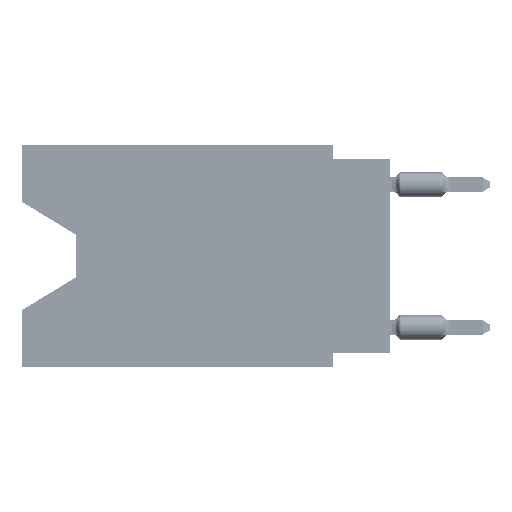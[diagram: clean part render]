
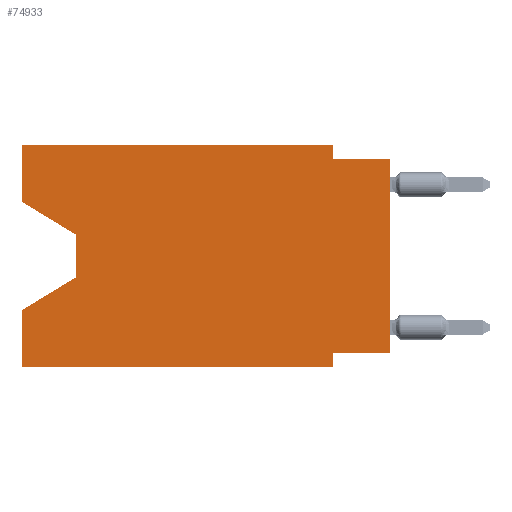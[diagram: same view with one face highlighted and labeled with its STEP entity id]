
A CAD part, left-side view. The second image highlights one B-rep face of the part: STEP entity #74933.
In plain terms, the highlighted planar face has unit normal (-1, 0, 0).
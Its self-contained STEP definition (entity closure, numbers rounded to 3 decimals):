
#1643 = ORIENTED_EDGE ( 'NONE', *, *, #59581, .T. ) ;
#3767 = CARTESIAN_POINT ( 'NONE',  ( 0., 13.97, -4.013 ) ) ;
#3869 = CARTESIAN_POINT ( 'NONE',  ( 0., 13.97, -5.893 ) ) ;
#3944 = VERTEX_POINT ( 'NONE', #62409 ) ;
#4007 = VERTEX_POINT ( 'NONE', #27999 ) ;
#4010 = VECTOR ( 'NONE', #70191, 1000. ) ;
#4307 = ORIENTED_EDGE ( 'NONE', *, *, #34257, .T. ) ;
#4495 = ORIENTED_EDGE ( 'NONE', *, *, #72244, .F. ) ;
#5738 = DIRECTION ( 'NONE',  ( 0., 1., 0. ) ) ;
#5944 = ORIENTED_EDGE ( 'NONE', *, *, #39216, .T. ) ;
#6484 = CARTESIAN_POINT ( 'NONE',  ( 0., 0., -9.271 ) ) ;
#7124 = ORIENTED_EDGE ( 'NONE', *, *, #42013, .F. ) ;
#7184 = PLANE ( 'NONE',  #61906 ) ;
#7588 = VECTOR ( 'NONE', #34961, 1000. ) ;
#7641 = DIRECTION ( 'NONE',  ( 0., -0.855, -0.519 ) ) ;
#9829 = VECTOR ( 'NONE', #7641, 1000. ) ;
#9914 = VERTEX_POINT ( 'NONE', #3767 ) ;
#10102 = ORIENTED_EDGE ( 'NONE', *, *, #59557, .F. ) ;
#10778 = CARTESIAN_POINT ( 'NONE',  ( 0., 2.54, -9.271 ) ) ;
#11284 = EDGE_CURVE ( 'NONE', #56904, #65937, #42937, .T. ) ;
#11451 = CARTESIAN_POINT ( 'NONE',  ( 0., 2.54, 0. ) ) ;
#12193 = ORIENTED_EDGE ( 'NONE', *, *, #66778, .F. ) ;
#13023 = DIRECTION ( 'NONE',  ( 0., -1., 0. ) ) ;
#14417 = CARTESIAN_POINT ( 'NONE',  ( 0., 16.383, 0. ) ) ;
#15063 = CARTESIAN_POINT ( 'NONE',  ( 0., 16.383, 0. ) ) ;
#16165 = LINE ( 'NONE', #58959, #32731 ) ;
#17858 = LINE ( 'NONE', #11451, #47762 ) ;
#19042 = LINE ( 'NONE', #67795, #57988 ) ;
#21041 = DIRECTION ( 'NONE',  ( 0., -1., 0. ) ) ;
#22310 = CARTESIAN_POINT ( 'NONE',  ( 0., 2.54, 0. ) ) ;
#24592 = VERTEX_POINT ( 'NONE', #46143 ) ;
#24802 = DIRECTION ( 'NONE',  ( 0., 0., -1. ) ) ;
#24850 = VERTEX_POINT ( 'NONE', #26475 ) ;
#25269 = VERTEX_POINT ( 'NONE', #62284 ) ;
#26475 = CARTESIAN_POINT ( 'NONE',  ( 0., 16.383, -2.546 ) ) ;
#27052 = EDGE_CURVE ( 'NONE', #24850, #25269, #40960, .T. ) ;
#27944 = CARTESIAN_POINT ( 'NONE',  ( 0., 0., -0.635 ) ) ;
#27999 = CARTESIAN_POINT ( 'NONE',  ( 0., 0., -0.635 ) ) ;
#28840 = CARTESIAN_POINT ( 'NONE',  ( 0., 2.54, -9.906 ) ) ;
#30872 = VERTEX_POINT ( 'NONE', #74119 ) ;
#31520 = CARTESIAN_POINT ( 'NONE',  ( 0., 13.97, -4.013 ) ) ;
#32284 = LINE ( 'NONE', #15063, #56442 ) ;
#32670 = LINE ( 'NONE', #31520, #69686 ) ;
#32731 = VECTOR ( 'NONE', #70539, 1000. ) ;
#32813 = ORIENTED_EDGE ( 'NONE', *, *, #77363, .T. ) ;
#32839 = LINE ( 'NONE', #14417, #78806 ) ;
#33634 = VERTEX_POINT ( 'NONE', #28840 ) ;
#34257 = EDGE_CURVE ( 'NONE', #9914, #63032, #32670, .T. ) ;
#34961 = DIRECTION ( 'NONE',  ( 0., 0., 1. ) ) ;
#35899 = VERTEX_POINT ( 'NONE', #22310 ) ;
#36657 = DIRECTION ( 'NONE',  ( 0., 0., -1. ) ) ;
#36780 = ORIENTED_EDGE ( 'NONE', *, *, #63275, .F. ) ;
#37490 = VECTOR ( 'NONE', #5738, 1000. ) ;
#38815 = DIRECTION ( 'NONE',  ( 0., 0., 1. ) ) ;
#39216 = EDGE_CURVE ( 'NONE', #63032, #24592, #58665, .T. ) ;
#40960 = LINE ( 'NONE', #65336, #7588 ) ;
#42013 = EDGE_CURVE ( 'NONE', #25269, #35899, #32284, .T. ) ;
#42151 = VECTOR ( 'NONE', #69914, 1000. ) ;
#42937 = LINE ( 'NONE', #66529, #37490 ) ;
#46143 = CARTESIAN_POINT ( 'NONE',  ( 0., 16.383, -7.36 ) ) ;
#46328 = LINE ( 'NONE', #27944, #42151 ) ;
#47762 = VECTOR ( 'NONE', #36657, 1000. ) ;
#49720 = EDGE_CURVE ( 'NONE', #3944, #33634, #19042, .T. ) ;
#55583 = FACE_OUTER_BOUND ( 'NONE', #58093, .T. ) ;
#56442 = VECTOR ( 'NONE', #21041, 1000. ) ;
#56891 = ORIENTED_EDGE ( 'NONE', *, *, #49720, .T. ) ;
#56904 = VERTEX_POINT ( 'NONE', #6484 ) ;
#57058 = DIRECTION ( 'NONE',  ( 0., 0., -1. ) ) ;
#57231 = CARTESIAN_POINT ( 'NONE',  ( 0., 16.383, -2.546 ) ) ;
#57988 = VECTOR ( 'NONE', #13023, 1000. ) ;
#58093 = EDGE_LOOP ( 'NONE', ( #1643, #4307, #5944, #10102, #56891, #12193, #66478, #32813, #36780, #4495, #7124, #60650 ) ) ;
#58213 = CARTESIAN_POINT ( 'NONE',  ( 0., 2.54, -9.906 ) ) ;
#58665 = LINE ( 'NONE', #3869, #73938 ) ;
#58959 = CARTESIAN_POINT ( 'NONE',  ( 0., 0., 0. ) ) ;
#59557 = EDGE_CURVE ( 'NONE', #3944, #24592, #32839, .T. ) ;
#59581 = EDGE_CURVE ( 'NONE', #24850, #9914, #62056, .T. ) ;
#60650 = ORIENTED_EDGE ( 'NONE', *, *, #27052, .F. ) ;
#61598 = DIRECTION ( 'NONE',  ( 1., 0., 0. ) ) ;
#61906 = AXIS2_PLACEMENT_3D ( 'NONE', #73980, #61598, #24802 ) ;
#62056 = LINE ( 'NONE', #57231, #9829 ) ;
#62284 = CARTESIAN_POINT ( 'NONE',  ( 0., 16.383, 0. ) ) ;
#62409 = CARTESIAN_POINT ( 'NONE',  ( 0., 16.383, -9.906 ) ) ;
#63032 = VERTEX_POINT ( 'NONE', #78787 ) ;
#63275 = EDGE_CURVE ( 'NONE', #30872, #4007, #46328, .T. ) ;
#65336 = CARTESIAN_POINT ( 'NONE',  ( 0., 16.383, 0. ) ) ;
#65937 = VERTEX_POINT ( 'NONE', #10778 ) ;
#66478 = ORIENTED_EDGE ( 'NONE', *, *, #11284, .F. ) ;
#66529 = CARTESIAN_POINT ( 'NONE',  ( 0., 0., -9.271 ) ) ;
#66778 = EDGE_CURVE ( 'NONE', #65937, #33634, #69791, .T. ) ;
#67795 = CARTESIAN_POINT ( 'NONE',  ( 0., 16.383, -9.906 ) ) ;
#69686 = VECTOR ( 'NONE', #57058, 1000. ) ;
#69791 = LINE ( 'NONE', #58213, #4010 ) ;
#69914 = DIRECTION ( 'NONE',  ( 0., -1., 0. ) ) ;
#70191 = DIRECTION ( 'NONE',  ( 0., 0., -1. ) ) ;
#70539 = DIRECTION ( 'NONE',  ( 0., 0., 1. ) ) ;
#72244 = EDGE_CURVE ( 'NONE', #35899, #30872, #17858, .T. ) ;
#73938 = VECTOR ( 'NONE', #76640, 1000. ) ;
#73980 = CARTESIAN_POINT ( 'NONE',  ( 0., 16.383, 0. ) ) ;
#74119 = CARTESIAN_POINT ( 'NONE',  ( 0., 2.54, -0.635 ) ) ;
#74933 = ADVANCED_FACE ( 'NONE', ( #55583 ), #7184, .F. ) ;
#76640 = DIRECTION ( 'NONE',  ( 0., 0.855, -0.519 ) ) ;
#77363 = EDGE_CURVE ( 'NONE', #56904, #4007, #16165, .T. ) ;
#78787 = CARTESIAN_POINT ( 'NONE',  ( 0., 13.97, -5.893 ) ) ;
#78806 = VECTOR ( 'NONE', #38815, 1000. ) ;
